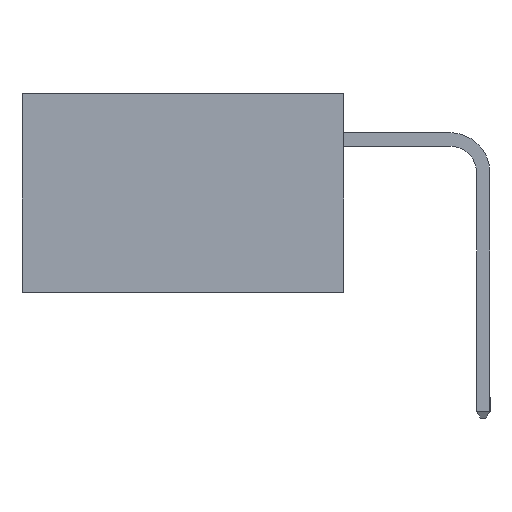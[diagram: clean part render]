
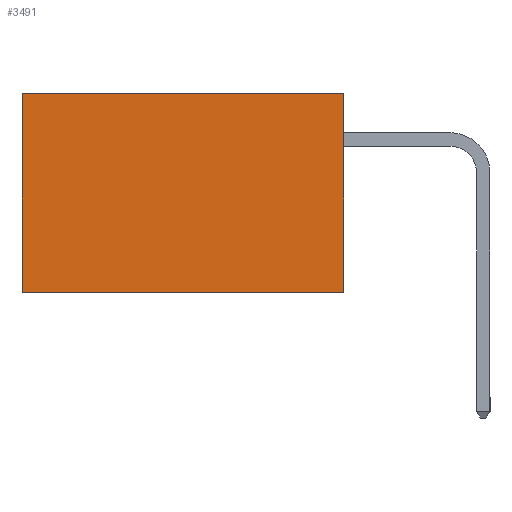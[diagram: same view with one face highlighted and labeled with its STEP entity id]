
A CAD part, left-side view. The second image highlights one B-rep face of the part: STEP entity #3491.
In plain terms, the highlighted planar face has unit normal (-1, 0, 0).
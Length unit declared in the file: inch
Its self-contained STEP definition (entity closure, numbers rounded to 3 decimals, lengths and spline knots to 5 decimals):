
#322 = LINE ( 'NONE', #10581, #9130 ) ;
#456 = DIRECTION ( 'NONE',  ( 0., 1., 0. ) ) ;
#904 = VERTEX_POINT ( 'NONE', #14415 ) ;
#2021 = EDGE_CURVE ( 'NONE', #10943, #13614, #16736, .T. ) ;
#2083 = VECTOR ( 'NONE', #14493, 39.37008 ) ;
#2921 = DIRECTION ( 'NONE',  ( 0., 0., -1. ) ) ;
#2927 = DIRECTION ( 'NONE',  ( 0., 0., -1. ) ) ;
#2995 = DIRECTION ( 'NONE',  ( 1., 0., 0. ) ) ;
#3174 = CARTESIAN_POINT ( 'NONE',  ( 0.2615, 0., -0.37 ) ) ;
#3221 = PLANE ( 'NONE',  #3335 ) ;
#3335 = AXIS2_PLACEMENT_3D ( 'NONE', #3174, #2995, #2921 ) ;
#3491 = ADVANCED_FACE ( 'NONE', ( #17788 ), #3221, .F. ) ;
#4692 = ORIENTED_EDGE ( 'NONE', *, *, #11138, .T. ) ;
#6389 = CARTESIAN_POINT ( 'NONE',  ( 0.2615, 0., -0.37 ) ) ;
#7619 = CARTESIAN_POINT ( 'NONE',  ( 0.2615, 0., 0. ) ) ;
#7725 = ORIENTED_EDGE ( 'NONE', *, *, #18266, .F. ) ;
#7859 = VECTOR ( 'NONE', #456, 39.37008 ) ;
#9016 = VERTEX_POINT ( 'NONE', #7619 ) ;
#9130 = VECTOR ( 'NONE', #10558, 39.37008 ) ;
#10558 = DIRECTION ( 'NONE',  ( 0., 0., -1. ) ) ;
#10581 = CARTESIAN_POINT ( 'NONE',  ( 0.2615, 0.6, -0.37 ) ) ;
#10943 = VERTEX_POINT ( 'NONE', #14099 ) ;
#11138 = EDGE_CURVE ( 'NONE', #904, #13614, #322, .T. ) ;
#11194 = CARTESIAN_POINT ( 'NONE',  ( 0.2615, 0., -0.37 ) ) ;
#12289 = VECTOR ( 'NONE', #2927, 39.37008 ) ;
#12828 = CARTESIAN_POINT ( 'NONE',  ( 0.2615, 0., 0. ) ) ;
#13614 = VERTEX_POINT ( 'NONE', #14902 ) ;
#13930 = ORIENTED_EDGE ( 'NONE', *, *, #18744, .T. ) ;
#14099 = CARTESIAN_POINT ( 'NONE',  ( 0.2615, 0., -0.37 ) ) ;
#14415 = CARTESIAN_POINT ( 'NONE',  ( 0.2615, 0.6, 0. ) ) ;
#14493 = DIRECTION ( 'NONE',  ( 0., 1., 0. ) ) ;
#14902 = CARTESIAN_POINT ( 'NONE',  ( 0.2615, 0.6, -0.37 ) ) ;
#15737 = LINE ( 'NONE', #12828, #2083 ) ;
#16613 = LINE ( 'NONE', #6389, #12289 ) ;
#16736 = LINE ( 'NONE', #11194, #7859 ) ;
#16737 = ORIENTED_EDGE ( 'NONE', *, *, #2021, .F. ) ;
#16828 = EDGE_LOOP ( 'NONE', ( #4692, #16737, #7725, #13930 ) ) ;
#17788 = FACE_OUTER_BOUND ( 'NONE', #16828, .T. ) ;
#18266 = EDGE_CURVE ( 'NONE', #9016, #10943, #16613, .T. ) ;
#18744 = EDGE_CURVE ( 'NONE', #9016, #904, #15737, .T. ) ;
